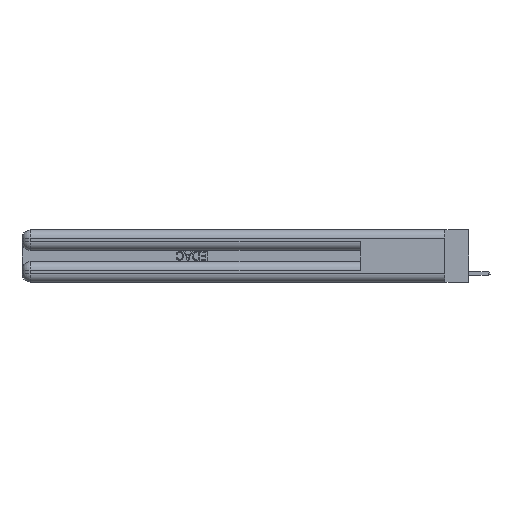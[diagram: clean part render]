
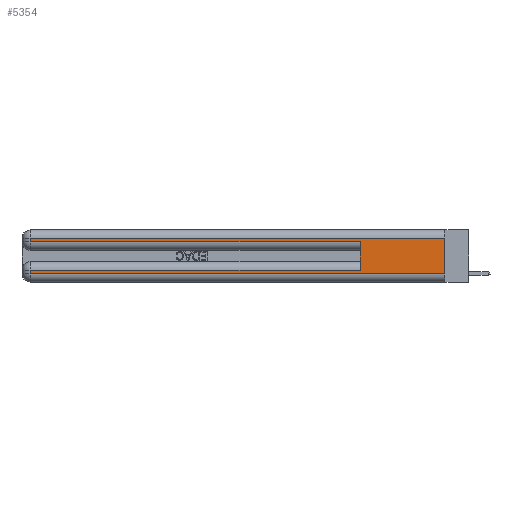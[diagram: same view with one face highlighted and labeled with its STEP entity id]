
A CAD part, left-side view. The second image highlights one B-rep face of the part: STEP entity #5354.
In plain terms, the highlighted planar face has unit normal (-1, 0, 0).
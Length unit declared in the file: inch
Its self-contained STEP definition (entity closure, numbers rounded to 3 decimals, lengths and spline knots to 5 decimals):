
#14 = VERTEX_POINT ( 'NONE', #2991 ) ;
#62 = CARTESIAN_POINT ( 'NONE',  ( 0., 2.94, 0.06 ) ) ;
#779 = DIRECTION ( 'NONE',  ( 0., 1., 0. ) ) ;
#1803 = LINE ( 'NONE', #23035, #12899 ) ;
#2154 = CARTESIAN_POINT ( 'NONE',  ( 0., 2.94, 0.31 ) ) ;
#2476 = ORIENTED_EDGE ( 'NONE', *, *, #11562, .T. ) ;
#2650 = VECTOR ( 'NONE', #779, 39.37008 ) ;
#2679 = CARTESIAN_POINT ( 'NONE',  ( 0., 2.94, 0.37 ) ) ;
#2684 = VECTOR ( 'NONE', #22400, 39.37008 ) ;
#2833 = LINE ( 'NONE', #2679, #23545 ) ;
#2991 = CARTESIAN_POINT ( 'NONE',  ( 0., 2.94, 0.285 ) ) ;
#3149 = EDGE_CURVE ( 'NONE', #15681, #17772, #24590, .T. ) ;
#3195 = CARTESIAN_POINT ( 'NONE',  ( 0., 0., 0.37 ) ) ;
#3458 = EDGE_LOOP ( 'NONE', ( #13566, #13896, #2476, #20706, #12675, #27768, #15398, #13477 ) ) ;
#5048 = AXIS2_PLACEMENT_3D ( 'NONE', #25130, #8119, #27474 ) ;
#5103 = DIRECTION ( 'NONE',  ( 0., -1., 0. ) ) ;
#5354 = ADVANCED_FACE ( 'NONE', ( #8264 ), #24975, .F. ) ;
#5415 = CARTESIAN_POINT ( 'NONE',  ( 0., 0., 0.285 ) ) ;
#5450 = LINE ( 'NONE', #14966, #2650 ) ;
#5642 = CARTESIAN_POINT ( 'NONE',  ( 0., 2.94, 0.085 ) ) ;
#5857 = CARTESIAN_POINT ( 'NONE',  ( 0., 0., 0.085 ) ) ;
#6868 = VECTOR ( 'NONE', #5103, 39.37008 ) ;
#6988 = EDGE_CURVE ( 'NONE', #15681, #19064, #5450, .T. ) ;
#8119 = DIRECTION ( 'NONE',  ( 1., 0., 0. ) ) ;
#8200 = LINE ( 'NONE', #5857, #2684 ) ;
#8264 = FACE_OUTER_BOUND ( 'NONE', #3458, .T. ) ;
#9848 = DIRECTION ( 'NONE',  ( 0., 0., -1. ) ) ;
#9896 = EDGE_CURVE ( 'NONE', #18824, #25261, #8200, .T. ) ;
#10981 = CARTESIAN_POINT ( 'NONE',  ( 0., 0., 0.06 ) ) ;
#11352 = EDGE_CURVE ( 'NONE', #29301, #17772, #12140, .T. ) ;
#11562 = EDGE_CURVE ( 'NONE', #19064, #14, #18190, .T. ) ;
#12140 = LINE ( 'NONE', #13853, #13194 ) ;
#12247 = VECTOR ( 'NONE', #18034, 39.37008 ) ;
#12675 = ORIENTED_EDGE ( 'NONE', *, *, #17462, .F. ) ;
#12715 = DIRECTION ( 'NONE',  ( 0., 0., -1. ) ) ;
#12899 = VECTOR ( 'NONE', #20998, 39.37008 ) ;
#13194 = VECTOR ( 'NONE', #23383, 39.37008 ) ;
#13477 = ORIENTED_EDGE ( 'NONE', *, *, #11352, .T. ) ;
#13566 = ORIENTED_EDGE ( 'NONE', *, *, #3149, .F. ) ;
#13853 = CARTESIAN_POINT ( 'NONE',  ( 0., 0., 0.06 ) ) ;
#13896 = ORIENTED_EDGE ( 'NONE', *, *, #6988, .T. ) ;
#14966 = CARTESIAN_POINT ( 'NONE',  ( 0., 0., 0.31 ) ) ;
#15398 = ORIENTED_EDGE ( 'NONE', *, *, #29837, .T. ) ;
#15681 = VERTEX_POINT ( 'NONE', #29361 ) ;
#17462 = EDGE_CURVE ( 'NONE', #18824, #26426, #1803, .T. ) ;
#17772 = VERTEX_POINT ( 'NONE', #10981 ) ;
#18034 = DIRECTION ( 'NONE',  ( 0., 0., -1. ) ) ;
#18190 = LINE ( 'NONE', #23033, #12247 ) ;
#18824 = VERTEX_POINT ( 'NONE', #28668 ) ;
#19064 = VERTEX_POINT ( 'NONE', #2154 ) ;
#19839 = CARTESIAN_POINT ( 'NONE',  ( 0., 0.6, 0.285 ) ) ;
#20706 = ORIENTED_EDGE ( 'NONE', *, *, #23147, .T. ) ;
#20998 = DIRECTION ( 'NONE',  ( 0., 0., 1. ) ) ;
#22400 = DIRECTION ( 'NONE',  ( 0., 1., 0. ) ) ;
#23033 = CARTESIAN_POINT ( 'NONE',  ( 0., 2.94, 0.37 ) ) ;
#23035 = CARTESIAN_POINT ( 'NONE',  ( 0., 0.6, 0.145 ) ) ;
#23147 = EDGE_CURVE ( 'NONE', #14, #26426, #23991, .T. ) ;
#23383 = DIRECTION ( 'NONE',  ( 0., -1., 0. ) ) ;
#23545 = VECTOR ( 'NONE', #9848, 39.37008 ) ;
#23991 = LINE ( 'NONE', #5415, #6868 ) ;
#24590 = LINE ( 'NONE', #3195, #24767 ) ;
#24767 = VECTOR ( 'NONE', #12715, 39.37008 ) ;
#24975 = PLANE ( 'NONE',  #5048 ) ;
#25130 = CARTESIAN_POINT ( 'NONE',  ( 0., 0., 0.37 ) ) ;
#25261 = VERTEX_POINT ( 'NONE', #5642 ) ;
#26426 = VERTEX_POINT ( 'NONE', #19839 ) ;
#27474 = DIRECTION ( 'NONE',  ( 0., 0., -1. ) ) ;
#27768 = ORIENTED_EDGE ( 'NONE', *, *, #9896, .T. ) ;
#28668 = CARTESIAN_POINT ( 'NONE',  ( 0., 0.6, 0.085 ) ) ;
#29301 = VERTEX_POINT ( 'NONE', #62 ) ;
#29361 = CARTESIAN_POINT ( 'NONE',  ( 0., 0., 0.31 ) ) ;
#29837 = EDGE_CURVE ( 'NONE', #25261, #29301, #2833, .T. ) ;
